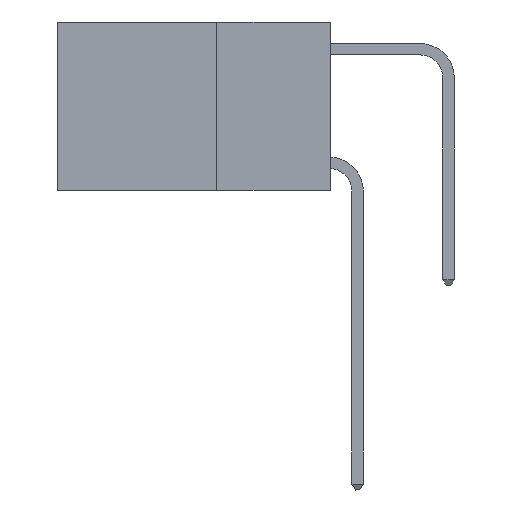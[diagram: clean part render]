
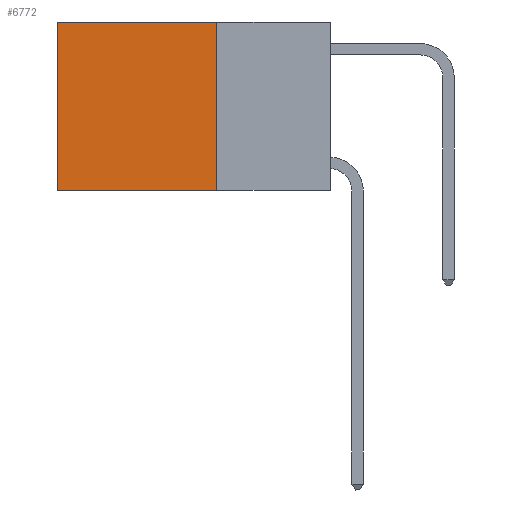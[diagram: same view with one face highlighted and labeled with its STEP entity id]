
A CAD part, left-side view. The second image highlights one B-rep face of the part: STEP entity #6772.
In plain terms, the highlighted planar face has unit normal (-1, 0, 0).
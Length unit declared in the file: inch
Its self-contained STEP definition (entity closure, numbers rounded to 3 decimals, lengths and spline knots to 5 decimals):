
#310 = VECTOR ( 'NONE', #30336, 39.37008 ) ;
#476 = EDGE_CURVE ( 'NONE', #22971, #31905, #17095, .T. ) ;
#940 = ORIENTED_EDGE ( 'NONE', *, *, #476, .F. ) ;
#2024 = VECTOR ( 'NONE', #18843, 39.37008 ) ;
#6772 = ADVANCED_FACE ( 'NONE', ( #13695 ), #32372, .F. ) ;
#7373 = VERTEX_POINT ( 'NONE', #19383 ) ;
#7573 = EDGE_CURVE ( 'NONE', #7373, #20727, #20843, .T. ) ;
#8623 = CARTESIAN_POINT ( 'NONE',  ( 0.2625, 0.25, -0.37 ) ) ;
#11548 = EDGE_LOOP ( 'NONE', ( #22544, #21923, #940, #17994 ) ) ;
#12030 = CARTESIAN_POINT ( 'NONE',  ( 0.2625, 0.25, 0. ) ) ;
#12230 = CARTESIAN_POINT ( 'NONE',  ( 0.2625, 0.6, 0. ) ) ;
#12346 = DIRECTION ( 'NONE',  ( 0., 0., -1. ) ) ;
#13357 = AXIS2_PLACEMENT_3D ( 'NONE', #14549, #32472, #17161 ) ;
#13695 = FACE_OUTER_BOUND ( 'NONE', #11548, .T. ) ;
#14129 = LINE ( 'NONE', #27737, #310 ) ;
#14549 = CARTESIAN_POINT ( 'NONE',  ( 0.2625, 0.25, 0. ) ) ;
#16246 = CARTESIAN_POINT ( 'NONE',  ( 0.2625, 0.25, 0. ) ) ;
#16289 = VECTOR ( 'NONE', #17156, 39.37008 ) ;
#17095 = LINE ( 'NONE', #12030, #16289 ) ;
#17156 = DIRECTION ( 'NONE',  ( 0., 0., -1. ) ) ;
#17161 = DIRECTION ( 'NONE',  ( 0., 0., -1. ) ) ;
#17994 = ORIENTED_EDGE ( 'NONE', *, *, #23555, .T. ) ;
#18843 = DIRECTION ( 'NONE',  ( 0., 1., 0. ) ) ;
#19242 = VECTOR ( 'NONE', #12346, 39.37008 ) ;
#19319 = CARTESIAN_POINT ( 'NONE',  ( 0.2625, 0.25, 0. ) ) ;
#19383 = CARTESIAN_POINT ( 'NONE',  ( 0.2625, 0.6, 0. ) ) ;
#20727 = VERTEX_POINT ( 'NONE', #26160 ) ;
#20843 = LINE ( 'NONE', #12230, #19242 ) ;
#21923 = ORIENTED_EDGE ( 'NONE', *, *, #30170, .F. ) ;
#22544 = ORIENTED_EDGE ( 'NONE', *, *, #7573, .T. ) ;
#22971 = VERTEX_POINT ( 'NONE', #19319 ) ;
#23455 = LINE ( 'NONE', #16246, #2024 ) ;
#23555 = EDGE_CURVE ( 'NONE', #22971, #7373, #23455, .T. ) ;
#26160 = CARTESIAN_POINT ( 'NONE',  ( 0.2625, 0.6, -0.37 ) ) ;
#27737 = CARTESIAN_POINT ( 'NONE',  ( 0.2625, 0.25, -0.37 ) ) ;
#30170 = EDGE_CURVE ( 'NONE', #31905, #20727, #14129, .T. ) ;
#30336 = DIRECTION ( 'NONE',  ( 0., 1., 0. ) ) ;
#31905 = VERTEX_POINT ( 'NONE', #8623 ) ;
#32372 = PLANE ( 'NONE',  #13357 ) ;
#32472 = DIRECTION ( 'NONE',  ( 1., 0., 0. ) ) ;
